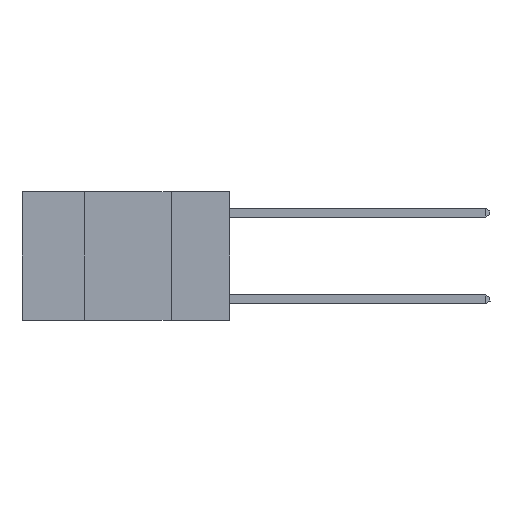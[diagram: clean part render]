
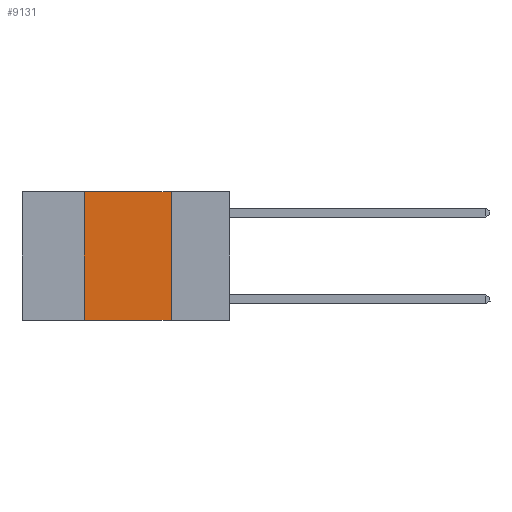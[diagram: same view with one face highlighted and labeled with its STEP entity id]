
A CAD part, left-side view. The second image highlights one B-rep face of the part: STEP entity #9131.
In plain terms, the highlighted planar face has unit normal (-1, 0, 0).
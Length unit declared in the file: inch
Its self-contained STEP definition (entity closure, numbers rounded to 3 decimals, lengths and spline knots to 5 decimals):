
#372 = DIRECTION ( 'NONE',  ( 0., 0., -1. ) ) ;
#525 = EDGE_LOOP ( 'NONE', ( #10411, #7427, #9715, #8614 ) ) ;
#728 = VECTOR ( 'NONE', #2978, 39.37008 ) ;
#1035 = VERTEX_POINT ( 'NONE', #4959 ) ;
#1249 = CARTESIAN_POINT ( 'NONE',  ( 0., 0.17, 0. ) ) ;
#1966 = EDGE_CURVE ( 'NONE', #1035, #4486, #6013, .T. ) ;
#2229 = VERTEX_POINT ( 'NONE', #8925 ) ;
#2978 = DIRECTION ( 'NONE',  ( 0., -1., 0. ) ) ;
#2998 = DIRECTION ( 'NONE',  ( 1., 0., 0. ) ) ;
#3258 = CARTESIAN_POINT ( 'NONE',  ( 0., 0.42, 0. ) ) ;
#3344 = LINE ( 'NONE', #1249, #5508 ) ;
#3841 = VECTOR ( 'NONE', #10307, 39.37008 ) ;
#4486 = VERTEX_POINT ( 'NONE', #6021 ) ;
#4775 = CARTESIAN_POINT ( 'NONE',  ( 0., 0.17, 0. ) ) ;
#4959 = CARTESIAN_POINT ( 'NONE',  ( 0., 0.42, -0.37 ) ) ;
#5013 = FACE_OUTER_BOUND ( 'NONE', #525, .T. ) ;
#5508 = VECTOR ( 'NONE', #372, 39.37008 ) ;
#5722 = DIRECTION ( 'NONE',  ( 0., 0., 1. ) ) ;
#6013 = LINE ( 'NONE', #9511, #3841 ) ;
#6021 = CARTESIAN_POINT ( 'NONE',  ( 0., 0.17, -0.37 ) ) ;
#6100 = VERTEX_POINT ( 'NONE', #4775 ) ;
#6600 = EDGE_CURVE ( 'NONE', #2229, #6100, #8065, .T. ) ;
#6681 = VECTOR ( 'NONE', #5722, 39.37008 ) ;
#7038 = CARTESIAN_POINT ( 'NONE',  ( 0., 0.6, 0. ) ) ;
#7427 = ORIENTED_EDGE ( 'NONE', *, *, #6600, .F. ) ;
#7755 = AXIS2_PLACEMENT_3D ( 'NONE', #10270, #2998, #8678 ) ;
#7875 = PLANE ( 'NONE',  #7755 ) ;
#8065 = LINE ( 'NONE', #7038, #728 ) ;
#8614 = ORIENTED_EDGE ( 'NONE', *, *, #1966, .T. ) ;
#8678 = DIRECTION ( 'NONE',  ( 0., 0., -1. ) ) ;
#8726 = EDGE_CURVE ( 'NONE', #1035, #2229, #9078, .T. ) ;
#8925 = CARTESIAN_POINT ( 'NONE',  ( 0., 0.42, 0. ) ) ;
#9076 = EDGE_CURVE ( 'NONE', #6100, #4486, #3344, .T. ) ;
#9078 = LINE ( 'NONE', #3258, #6681 ) ;
#9131 = ADVANCED_FACE ( 'NONE', ( #5013 ), #7875, .F. ) ;
#9511 = CARTESIAN_POINT ( 'NONE',  ( 0., 0.6, -0.37 ) ) ;
#9715 = ORIENTED_EDGE ( 'NONE', *, *, #8726, .F. ) ;
#10270 = CARTESIAN_POINT ( 'NONE',  ( 0., 0.6, 0. ) ) ;
#10307 = DIRECTION ( 'NONE',  ( 0., -1., 0. ) ) ;
#10411 = ORIENTED_EDGE ( 'NONE', *, *, #9076, .F. ) ;
